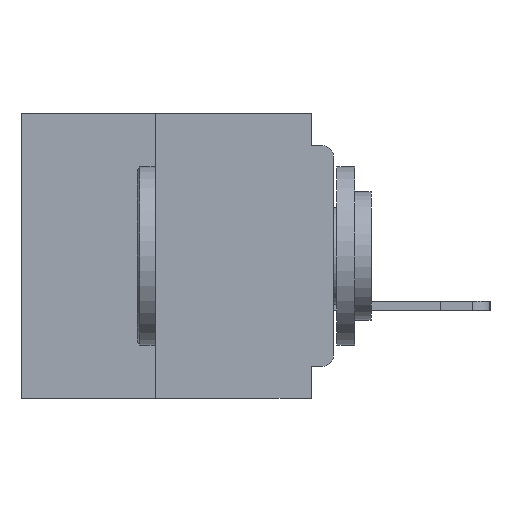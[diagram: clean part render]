
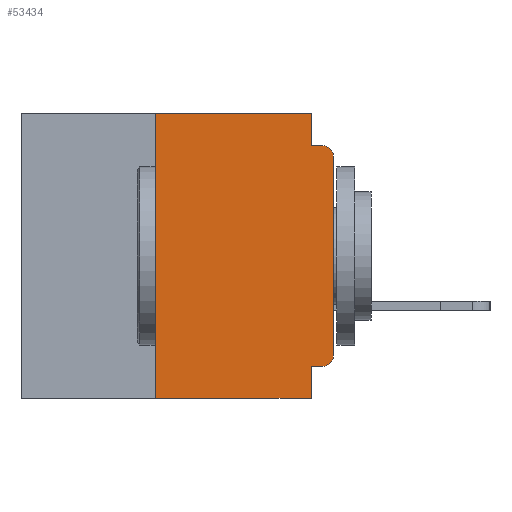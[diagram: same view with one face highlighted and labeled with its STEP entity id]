
A CAD part, left-side view. The second image highlights one B-rep face of the part: STEP entity #53434.
In plain terms, the highlighted planar face has unit normal (-1, 0, 0).
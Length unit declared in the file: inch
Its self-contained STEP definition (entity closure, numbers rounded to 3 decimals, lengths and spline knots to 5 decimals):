
#330 = VERTEX_POINT ( 'NONE', #53595 ) ;
#673 = EDGE_CURVE ( 'NONE', #27883, #61218, #31226, .T. ) ;
#1457 = CARTESIAN_POINT ( 'NONE',  ( 0., 0.015, -0.34 ) ) ;
#2287 = EDGE_CURVE ( 'NONE', #4321, #330, #40471, .T. ) ;
#2734 = CARTESIAN_POINT ( 'NONE',  ( 0., 0.25, -0.4 ) ) ;
#2980 = EDGE_CURVE ( 'NONE', #4321, #52984, #8165, .T. ) ;
#3363 = LINE ( 'NONE', #52791, #28527 ) ;
#3459 = ORIENTED_EDGE ( 'NONE', *, *, #2980, .F. ) ;
#4321 = VERTEX_POINT ( 'NONE', #2734 ) ;
#4638 = ORIENTED_EDGE ( 'NONE', *, *, #59430, .F. ) ;
#4776 = VERTEX_POINT ( 'NONE', #41181 ) ;
#4977 = EDGE_CURVE ( 'NONE', #52984, #17484, #30624, .T. ) ;
#6356 = ORIENTED_EDGE ( 'NONE', *, *, #4977, .F. ) ;
#6550 = DIRECTION ( 'NONE',  ( 0., 0., -1. ) ) ;
#6557 = VECTOR ( 'NONE', #28926, 39.37008 ) ;
#6955 = LINE ( 'NONE', #10665, #18742 ) ;
#8165 = LINE ( 'NONE', #28577, #6557 ) ;
#8552 = DIRECTION ( 'NONE',  ( -1., 0., 0. ) ) ;
#9260 = CARTESIAN_POINT ( 'NONE',  ( 0., 0., -0.355 ) ) ;
#10665 = CARTESIAN_POINT ( 'NONE',  ( 0., 0., 0. ) ) ;
#11109 = ORIENTED_EDGE ( 'NONE', *, *, #2287, .T. ) ;
#11742 = LINE ( 'NONE', #34728, #51860 ) ;
#13780 = VECTOR ( 'NONE', #55096, 39.37008 ) ;
#15012 = VERTEX_POINT ( 'NONE', #20169 ) ;
#15059 = ORIENTED_EDGE ( 'NONE', *, *, #53503, .F. ) ;
#17484 = VERTEX_POINT ( 'NONE', #49160 ) ;
#17657 = DIRECTION ( 'NONE',  ( 0., -1., 0. ) ) ;
#18742 = VECTOR ( 'NONE', #50890, 39.37008 ) ;
#19157 = PLANE ( 'NONE',  #45655 ) ;
#20169 = CARTESIAN_POINT ( 'NONE',  ( 0., 0., -0.06 ) ) ;
#20517 = CARTESIAN_POINT ( 'NONE',  ( 0., 0.25, 0. ) ) ;
#21146 = ORIENTED_EDGE ( 'NONE', *, *, #673, .F. ) ;
#22114 = CARTESIAN_POINT ( 'NONE',  ( 0., 0., -0.34 ) ) ;
#24150 = CARTESIAN_POINT ( 'NONE',  ( 0., 0.437, 0. ) ) ;
#24733 = CIRCLE ( 'NONE', #47090, 0.015 ) ;
#25226 = VERTEX_POINT ( 'NONE', #22114 ) ;
#27720 = CARTESIAN_POINT ( 'NONE',  ( 0., 0.437, 0. ) ) ;
#27883 = VERTEX_POINT ( 'NONE', #38880 ) ;
#28203 = EDGE_CURVE ( 'NONE', #4776, #25226, #45825, .T. ) ;
#28527 = VECTOR ( 'NONE', #57849, 39.37008 ) ;
#28577 = CARTESIAN_POINT ( 'NONE',  ( 0., 0.25, -0.4 ) ) ;
#28926 = DIRECTION ( 'NONE',  ( 0., 0., 1. ) ) ;
#29232 = DIRECTION ( 'NONE',  ( 1., 0., 0. ) ) ;
#29256 = ORIENTED_EDGE ( 'NONE', *, *, #28203, .T. ) ;
#30088 = CARTESIAN_POINT ( 'NONE',  ( 0., 0.015, -0.06 ) ) ;
#30624 = LINE ( 'NONE', #27720, #44024 ) ;
#31226 = LINE ( 'NONE', #46753, #43059 ) ;
#34728 = CARTESIAN_POINT ( 'NONE',  ( 0., 0.031, -0.4 ) ) ;
#35132 = DIRECTION ( 'NONE',  ( 0., 0., -1. ) ) ;
#36628 = DIRECTION ( 'NONE',  ( -1., 0., 0. ) ) ;
#38880 = CARTESIAN_POINT ( 'NONE',  ( 0., 0.031, -0.045 ) ) ;
#39468 = LINE ( 'NONE', #9260, #64607 ) ;
#40471 = LINE ( 'NONE', #56104, #13780 ) ;
#41181 = CARTESIAN_POINT ( 'NONE',  ( 0., 0.015, -0.355 ) ) ;
#41627 = FACE_OUTER_BOUND ( 'NONE', #50420, .T. ) ;
#42545 = AXIS2_PLACEMENT_3D ( 'NONE', #1457, #36628, #6550 ) ;
#43059 = VECTOR ( 'NONE', #46915, 39.37008 ) ;
#44024 = VECTOR ( 'NONE', #17657, 39.37008 ) ;
#45655 = AXIS2_PLACEMENT_3D ( 'NONE', #24150, #29232, #64402 ) ;
#45825 = CIRCLE ( 'NONE', #42545, 0.015 ) ;
#46534 = EDGE_CURVE ( 'NONE', #25226, #15012, #6955, .T. ) ;
#46753 = CARTESIAN_POINT ( 'NONE',  ( 0., 0., -0.045 ) ) ;
#46915 = DIRECTION ( 'NONE',  ( 0., -1., 0. ) ) ;
#47090 = AXIS2_PLACEMENT_3D ( 'NONE', #30088, #8552, #35132 ) ;
#47706 = ORIENTED_EDGE ( 'NONE', *, *, #51243, .F. ) ;
#47759 = ORIENTED_EDGE ( 'NONE', *, *, #46534, .T. ) ;
#49160 = CARTESIAN_POINT ( 'NONE',  ( 0., 0.031, 0. ) ) ;
#49439 = ORIENTED_EDGE ( 'NONE', *, *, #57734, .T. ) ;
#50420 = EDGE_LOOP ( 'NONE', ( #47759, #49439, #21146, #47706, #6356, #3459, #11109, #15059, #4638, #29256 ) ) ;
#50890 = DIRECTION ( 'NONE',  ( 0., 0., 1. ) ) ;
#51243 = EDGE_CURVE ( 'NONE', #17484, #27883, #3363, .T. ) ;
#51860 = VECTOR ( 'NONE', #64831, 39.37008 ) ;
#52791 = CARTESIAN_POINT ( 'NONE',  ( 0., 0.031, 0. ) ) ;
#52984 = VERTEX_POINT ( 'NONE', #20517 ) ;
#53434 = ADVANCED_FACE ( 'NONE', ( #41627 ), #19157, .F. ) ;
#53503 = EDGE_CURVE ( 'NONE', #64894, #330, #11742, .T. ) ;
#53595 = CARTESIAN_POINT ( 'NONE',  ( 0., 0.031, -0.4 ) ) ;
#55096 = DIRECTION ( 'NONE',  ( 0., -1., 0. ) ) ;
#56104 = CARTESIAN_POINT ( 'NONE',  ( 0., 0.437, -0.4 ) ) ;
#57365 = CARTESIAN_POINT ( 'NONE',  ( 0., 0.031, -0.355 ) ) ;
#57734 = EDGE_CURVE ( 'NONE', #15012, #61218, #24733, .T. ) ;
#57849 = DIRECTION ( 'NONE',  ( 0., 0., -1. ) ) ;
#58641 = CARTESIAN_POINT ( 'NONE',  ( 0., 0.015, -0.045 ) ) ;
#59430 = EDGE_CURVE ( 'NONE', #4776, #64894, #39468, .T. ) ;
#61218 = VERTEX_POINT ( 'NONE', #58641 ) ;
#64373 = DIRECTION ( 'NONE',  ( 0., 1., 0. ) ) ;
#64402 = DIRECTION ( 'NONE',  ( 0., 0., -1. ) ) ;
#64607 = VECTOR ( 'NONE', #64373, 39.37008 ) ;
#64831 = DIRECTION ( 'NONE',  ( 0., 0., -1. ) ) ;
#64894 = VERTEX_POINT ( 'NONE', #57365 ) ;
